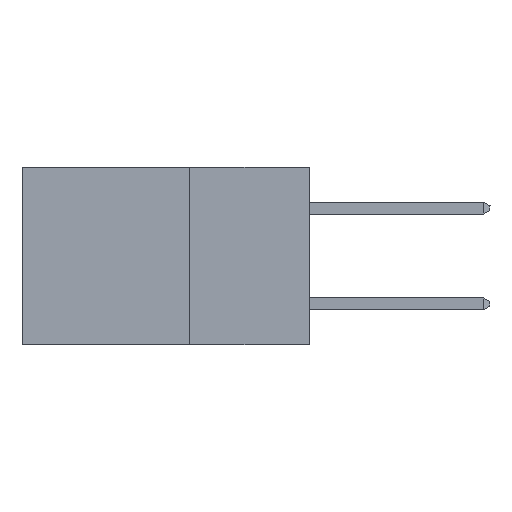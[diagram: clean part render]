
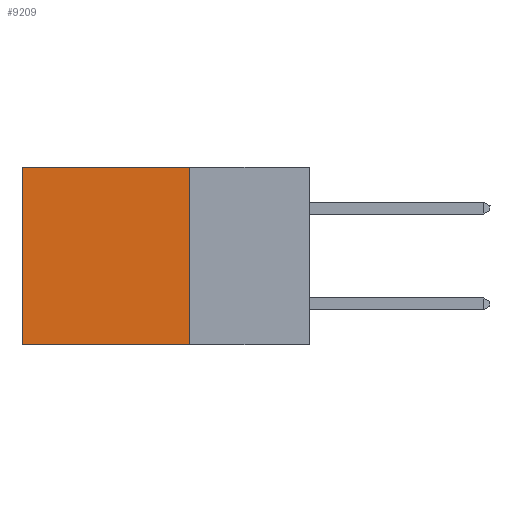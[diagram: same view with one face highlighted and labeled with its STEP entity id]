
A CAD part, left-side view. The second image highlights one B-rep face of the part: STEP entity #9209.
In plain terms, the highlighted planar face has unit normal (-1, 0, 0).
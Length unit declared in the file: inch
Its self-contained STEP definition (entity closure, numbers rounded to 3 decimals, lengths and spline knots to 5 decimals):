
#306 = LINE ( 'NONE', #10250, #17755 ) ;
#777 = PLANE ( 'NONE',  #10567 ) ;
#1289 = LINE ( 'NONE', #18706, #18709 ) ;
#1349 = CARTESIAN_POINT ( 'NONE',  ( 0.2875, 0.6, -0.37 ) ) ;
#1936 = VERTEX_POINT ( 'NONE', #1349 ) ;
#1987 = CARTESIAN_POINT ( 'NONE',  ( 0.2875, 0.25, 0. ) ) ;
#2521 = DIRECTION ( 'NONE',  ( 0., 0., -1. ) ) ;
#2762 = LINE ( 'NONE', #20847, #16113 ) ;
#3469 = EDGE_CURVE ( 'NONE', #15658, #1936, #306, .T. ) ;
#3525 = ORIENTED_EDGE ( 'NONE', *, *, #7777, .F. ) ;
#3541 = CARTESIAN_POINT ( 'NONE',  ( 0.2875, 0.25, -0.37 ) ) ;
#4049 = FACE_OUTER_BOUND ( 'NONE', #20660, .T. ) ;
#4757 = DIRECTION ( 'NONE',  ( 0., 1., 0. ) ) ;
#5436 = ORIENTED_EDGE ( 'NONE', *, *, #11335, .F. ) ;
#5766 = ORIENTED_EDGE ( 'NONE', *, *, #21768, .T. ) ;
#5937 = CARTESIAN_POINT ( 'NONE',  ( 0.2875, 0.25, 0. ) ) ;
#7777 = EDGE_CURVE ( 'NONE', #10618, #1936, #2762, .T. ) ;
#8003 = VECTOR ( 'NONE', #14112, 39.37008 ) ;
#9209 = ADVANCED_FACE ( 'NONE', ( #4049 ), #777, .F. ) ;
#9606 = LINE ( 'NONE', #1987, #8003 ) ;
#10250 = CARTESIAN_POINT ( 'NONE',  ( 0.2875, 0.6, 0. ) ) ;
#10275 = DIRECTION ( 'NONE',  ( 0., 0., -1. ) ) ;
#10398 = DIRECTION ( 'NONE',  ( 0., 1., 0. ) ) ;
#10567 = AXIS2_PLACEMENT_3D ( 'NONE', #5937, #12892, #2521 ) ;
#10618 = VERTEX_POINT ( 'NONE', #3541 ) ;
#10993 = VERTEX_POINT ( 'NONE', #21851 ) ;
#11252 = CARTESIAN_POINT ( 'NONE',  ( 0.2875, 0.6, 0. ) ) ;
#11335 = EDGE_CURVE ( 'NONE', #10993, #10618, #9606, .T. ) ;
#11631 = ORIENTED_EDGE ( 'NONE', *, *, #3469, .T. ) ;
#12892 = DIRECTION ( 'NONE',  ( 1., 0., 0. ) ) ;
#14112 = DIRECTION ( 'NONE',  ( 0., 0., -1. ) ) ;
#15658 = VERTEX_POINT ( 'NONE', #11252 ) ;
#16113 = VECTOR ( 'NONE', #10398, 39.37008 ) ;
#17755 = VECTOR ( 'NONE', #10275, 39.37008 ) ;
#18706 = CARTESIAN_POINT ( 'NONE',  ( 0.2875, 0.25, 0. ) ) ;
#18709 = VECTOR ( 'NONE', #4757, 39.37008 ) ;
#20660 = EDGE_LOOP ( 'NONE', ( #11631, #3525, #5436, #5766 ) ) ;
#20847 = CARTESIAN_POINT ( 'NONE',  ( 0.2875, 0.25, -0.37 ) ) ;
#21768 = EDGE_CURVE ( 'NONE', #10993, #15658, #1289, .T. ) ;
#21851 = CARTESIAN_POINT ( 'NONE',  ( 0.2875, 0.25, 0. ) ) ;
